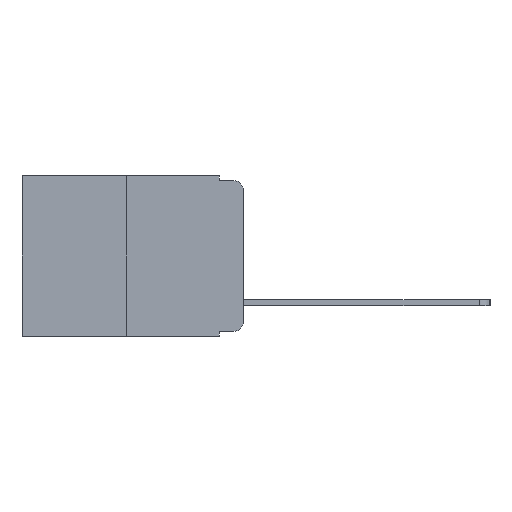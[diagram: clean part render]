
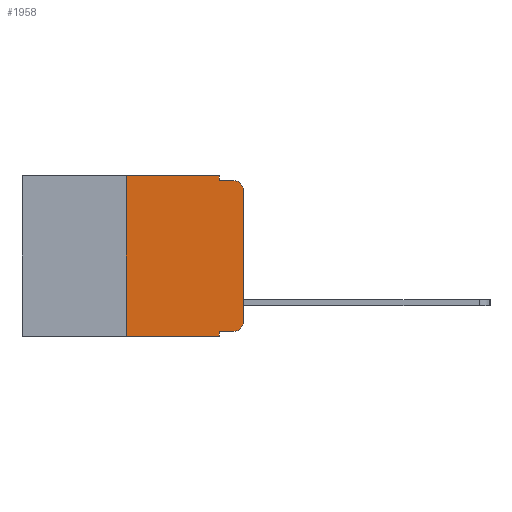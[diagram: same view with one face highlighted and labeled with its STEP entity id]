
A CAD part, left-side view. The second image highlights one B-rep face of the part: STEP entity #1958.
In plain terms, the highlighted planar face has unit normal (-1, 0, 0).
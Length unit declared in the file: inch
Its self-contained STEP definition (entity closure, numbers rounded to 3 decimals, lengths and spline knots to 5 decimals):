
#75 = VERTEX_POINT ( 'NONE', #2635 ) ;
#176 = EDGE_CURVE ( 'NONE', #4351, #5421, #9985, .T. ) ;
#335 = CARTESIAN_POINT ( 'NONE',  ( 0., 0., 0. ) ) ;
#484 = EDGE_CURVE ( 'NONE', #9441, #75, #3028, .T. ) ;
#557 = VERTEX_POINT ( 'NONE', #11138 ) ;
#702 = AXIS2_PLACEMENT_3D ( 'NONE', #8172, #9279, #9605 ) ;
#711 = CARTESIAN_POINT ( 'NONE',  ( 0., 0.051, 0. ) ) ;
#1223 = CARTESIAN_POINT ( 'NONE',  ( 0., 0.02, -0.333 ) ) ;
#1271 = VERTEX_POINT ( 'NONE', #711 ) ;
#1434 = FACE_OUTER_BOUND ( 'NONE', #6049, .T. ) ;
#1692 = VECTOR ( 'NONE', #10779, 39.37008 ) ;
#1958 = ADVANCED_FACE ( 'NONE', ( #1434 ), #7006, .F. ) ;
#2143 = CARTESIAN_POINT ( 'NONE',  ( 0., 0.051, -0.333 ) ) ;
#2180 = EDGE_CURVE ( 'NONE', #557, #9441, #6641, .T. ) ;
#2187 = VECTOR ( 'NONE', #4763, 39.37008 ) ;
#2332 = VECTOR ( 'NONE', #6831, 39.37008 ) ;
#2457 = EDGE_CURVE ( 'NONE', #7813, #75, #6245, .T. ) ;
#2635 = CARTESIAN_POINT ( 'NONE',  ( 0., 0.02, -0.01 ) ) ;
#2779 = EDGE_CURVE ( 'NONE', #4970, #7073, #9364, .T. ) ;
#3028 = CIRCLE ( 'NONE', #702, 0.02 ) ;
#3043 = EDGE_CURVE ( 'NONE', #6013, #557, #11203, .T. ) ;
#3044 = DIRECTION ( 'NONE',  ( 0., 0., -1. ) ) ;
#4340 = LINE ( 'NONE', #5185, #1692 ) ;
#4351 = VERTEX_POINT ( 'NONE', #9463 ) ;
#4620 = DIRECTION ( 'NONE',  ( 0., -1., 0. ) ) ;
#4763 = DIRECTION ( 'NONE',  ( 0., 0., 1. ) ) ;
#4807 = DIRECTION ( 'NONE',  ( 0., 0., 1. ) ) ;
#4823 = ORIENTED_EDGE ( 'NONE', *, *, #7152, .T. ) ;
#4859 = ORIENTED_EDGE ( 'NONE', *, *, #2779, .F. ) ;
#4970 = VERTEX_POINT ( 'NONE', #2143 ) ;
#5185 = CARTESIAN_POINT ( 'NONE',  ( 0., 0.051, -0.333 ) ) ;
#5189 = AXIS2_PLACEMENT_3D ( 'NONE', #7021, #7168, #3044 ) ;
#5254 = LINE ( 'NONE', #6239, #2332 ) ;
#5421 = VERTEX_POINT ( 'NONE', #10017 ) ;
#5462 = ORIENTED_EDGE ( 'NONE', *, *, #6040, .T. ) ;
#5739 = ORIENTED_EDGE ( 'NONE', *, *, #176, .F. ) ;
#5837 = DIRECTION ( 'NONE',  ( 0., -1., 0. ) ) ;
#5877 = CARTESIAN_POINT ( 'NONE',  ( 0., 0.051, -0.01 ) ) ;
#5964 = VECTOR ( 'NONE', #5837, 39.37008 ) ;
#5966 = ORIENTED_EDGE ( 'NONE', *, *, #7469, .F. ) ;
#5980 = CARTESIAN_POINT ( 'NONE',  ( 0., 0.051, 0. ) ) ;
#6013 = VERTEX_POINT ( 'NONE', #1223 ) ;
#6040 = EDGE_CURVE ( 'NONE', #4351, #7073, #5254, .T. ) ;
#6049 = EDGE_LOOP ( 'NONE', ( #8463, #7005, #11059, #6221, #5966, #5739, #5462, #4859, #4823, #11050 ) ) ;
#6221 = ORIENTED_EDGE ( 'NONE', *, *, #10249, .F. ) ;
#6238 = CARTESIAN_POINT ( 'NONE',  ( 0., 0.051, 0. ) ) ;
#6239 = CARTESIAN_POINT ( 'NONE',  ( 0., 0.473, -0.343 ) ) ;
#6245 = LINE ( 'NONE', #5877, #5964 ) ;
#6480 = DIRECTION ( 'NONE',  ( 0., 0., -1. ) ) ;
#6641 = LINE ( 'NONE', #335, #2187 ) ;
#6831 = DIRECTION ( 'NONE',  ( 0., -1., 0. ) ) ;
#6842 = DIRECTION ( 'NONE',  ( 0., 0., -1. ) ) ;
#7002 = DIRECTION ( 'NONE',  ( -1., 0., 0. ) ) ;
#7005 = ORIENTED_EDGE ( 'NONE', *, *, #484, .T. ) ;
#7006 = PLANE ( 'NONE',  #5189 ) ;
#7021 = CARTESIAN_POINT ( 'NONE',  ( 0., 0.473, 0. ) ) ;
#7073 = VERTEX_POINT ( 'NONE', #9972 ) ;
#7152 = EDGE_CURVE ( 'NONE', #4970, #6013, #4340, .T. ) ;
#7168 = DIRECTION ( 'NONE',  ( 1., 0., 0. ) ) ;
#7239 = LINE ( 'NONE', #6238, #9073 ) ;
#7261 = CARTESIAN_POINT ( 'NONE',  ( 0., 0.051, -0.01 ) ) ;
#7469 = EDGE_CURVE ( 'NONE', #5421, #1271, #10280, .T. ) ;
#7813 = VERTEX_POINT ( 'NONE', #7261 ) ;
#7870 = DIRECTION ( 'NONE',  ( 0., 0., -1. ) ) ;
#7939 = VECTOR ( 'NONE', #4807, 39.37008 ) ;
#8133 = CARTESIAN_POINT ( 'NONE',  ( 0., 0.02, -0.313 ) ) ;
#8172 = CARTESIAN_POINT ( 'NONE',  ( 0., 0.02, -0.03 ) ) ;
#8292 = AXIS2_PLACEMENT_3D ( 'NONE', #8133, #7002, #6480 ) ;
#8463 = ORIENTED_EDGE ( 'NONE', *, *, #2180, .T. ) ;
#8506 = VECTOR ( 'NONE', #4620, 39.37008 ) ;
#9073 = VECTOR ( 'NONE', #7870, 39.37008 ) ;
#9095 = CARTESIAN_POINT ( 'NONE',  ( 0., 0.25, 0. ) ) ;
#9279 = DIRECTION ( 'NONE',  ( -1., 0., 0. ) ) ;
#9332 = CARTESIAN_POINT ( 'NONE',  ( 0., 0., -0.03 ) ) ;
#9364 = LINE ( 'NONE', #5980, #11092 ) ;
#9441 = VERTEX_POINT ( 'NONE', #9332 ) ;
#9463 = CARTESIAN_POINT ( 'NONE',  ( 0., 0.25, -0.343 ) ) ;
#9605 = DIRECTION ( 'NONE',  ( 0., 0., -1. ) ) ;
#9971 = CARTESIAN_POINT ( 'NONE',  ( 0., 0.473, 0. ) ) ;
#9972 = CARTESIAN_POINT ( 'NONE',  ( 0., 0.051, -0.343 ) ) ;
#9985 = LINE ( 'NONE', #9095, #7939 ) ;
#10017 = CARTESIAN_POINT ( 'NONE',  ( 0., 0.25, 0. ) ) ;
#10249 = EDGE_CURVE ( 'NONE', #1271, #7813, #7239, .T. ) ;
#10280 = LINE ( 'NONE', #9971, #8506 ) ;
#10779 = DIRECTION ( 'NONE',  ( 0., -1., 0. ) ) ;
#11050 = ORIENTED_EDGE ( 'NONE', *, *, #3043, .T. ) ;
#11059 = ORIENTED_EDGE ( 'NONE', *, *, #2457, .F. ) ;
#11092 = VECTOR ( 'NONE', #6842, 39.37008 ) ;
#11138 = CARTESIAN_POINT ( 'NONE',  ( 0., 0., -0.313 ) ) ;
#11203 = CIRCLE ( 'NONE', #8292, 0.02 ) ;
